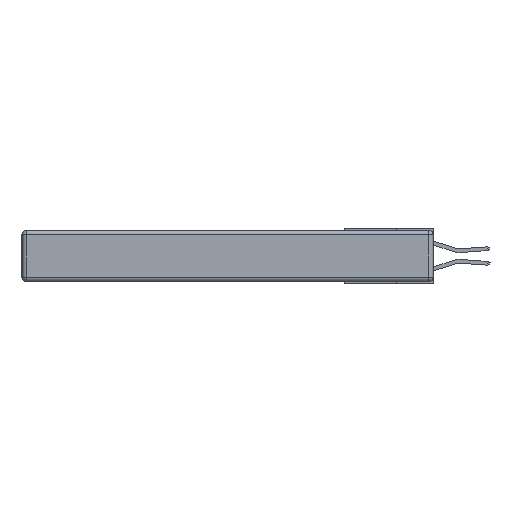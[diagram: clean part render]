
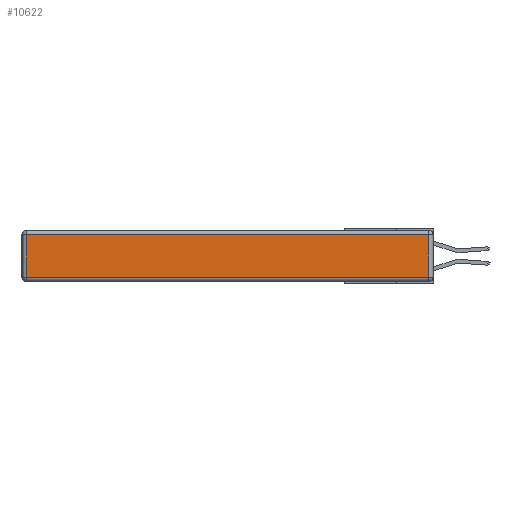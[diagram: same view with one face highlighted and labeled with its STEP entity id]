
A CAD part, left-side view. The second image highlights one B-rep face of the part: STEP entity #10622.
In plain terms, the highlighted planar face has unit normal (-1, 0, 0).
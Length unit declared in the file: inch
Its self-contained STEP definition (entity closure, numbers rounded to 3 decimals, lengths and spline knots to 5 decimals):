
#328 = VECTOR ( 'NONE', #13593, 39.37008 ) ;
#397 = VERTEX_POINT ( 'NONE', #6900 ) ;
#608 = FACE_OUTER_BOUND ( 'NONE', #4610, .T. ) ;
#765 = EDGE_CURVE ( 'NONE', #397, #18157, #17456, .T. ) ;
#3399 = CARTESIAN_POINT ( 'NONE',  ( 0., 0., -0.313 ) ) ;
#4228 = DIRECTION ( 'NONE',  ( 0., 1., 0. ) ) ;
#4439 = DIRECTION ( 'NONE',  ( -1., 0., 0. ) ) ;
#4610 = EDGE_LOOP ( 'NONE', ( #9265, #10805, #6260, #17234 ) ) ;
#4956 = CARTESIAN_POINT ( 'NONE',  ( 0., 0.03, -0.343 ) ) ;
#6260 = ORIENTED_EDGE ( 'NONE', *, *, #16778, .T. ) ;
#6520 = CARTESIAN_POINT ( 'NONE',  ( 0., 2.72, -0.343 ) ) ;
#6900 = CARTESIAN_POINT ( 'NONE',  ( 0., 2.72, -0.03 ) ) ;
#7521 = CARTESIAN_POINT ( 'NONE',  ( 0., 0., -0.343 ) ) ;
#8212 = PLANE ( 'NONE',  #15761 ) ;
#8270 = LINE ( 'NONE', #3399, #328 ) ;
#8598 = VECTOR ( 'NONE', #15369, 39.37008 ) ;
#8639 = CARTESIAN_POINT ( 'NONE',  ( 0., 0.03, -0.313 ) ) ;
#9265 = ORIENTED_EDGE ( 'NONE', *, *, #11455, .T. ) ;
#10438 = LINE ( 'NONE', #4956, #8598 ) ;
#10451 = VERTEX_POINT ( 'NONE', #8639 ) ;
#10622 = ADVANCED_FACE ( 'NONE', ( #608 ), #8212, .T. ) ;
#10805 = ORIENTED_EDGE ( 'NONE', *, *, #14598, .T. ) ;
#10882 = VECTOR ( 'NONE', #15361, 39.37008 ) ;
#11455 = EDGE_CURVE ( 'NONE', #18157, #10451, #8270, .T. ) ;
#11597 = CARTESIAN_POINT ( 'NONE',  ( 0., 2.75, -0.03 ) ) ;
#13361 = VECTOR ( 'NONE', #4228, 39.37008 ) ;
#13464 = CARTESIAN_POINT ( 'NONE',  ( 0., 2.72, -0.313 ) ) ;
#13593 = DIRECTION ( 'NONE',  ( 0., -1., 0. ) ) ;
#14598 = EDGE_CURVE ( 'NONE', #10451, #17420, #10438, .T. ) ;
#15361 = DIRECTION ( 'NONE',  ( 0., 0., -1. ) ) ;
#15369 = DIRECTION ( 'NONE',  ( 0., 0., 1. ) ) ;
#15657 = LINE ( 'NONE', #11597, #13361 ) ;
#15761 = AXIS2_PLACEMENT_3D ( 'NONE', #7521, #4439, #17850 ) ;
#16778 = EDGE_CURVE ( 'NONE', #17420, #397, #15657, .T. ) ;
#17234 = ORIENTED_EDGE ( 'NONE', *, *, #765, .T. ) ;
#17420 = VERTEX_POINT ( 'NONE', #19182 ) ;
#17456 = LINE ( 'NONE', #6520, #10882 ) ;
#17850 = DIRECTION ( 'NONE',  ( 0., 0., 1. ) ) ;
#18157 = VERTEX_POINT ( 'NONE', #13464 ) ;
#19182 = CARTESIAN_POINT ( 'NONE',  ( 0., 0.03, -0.03 ) ) ;
